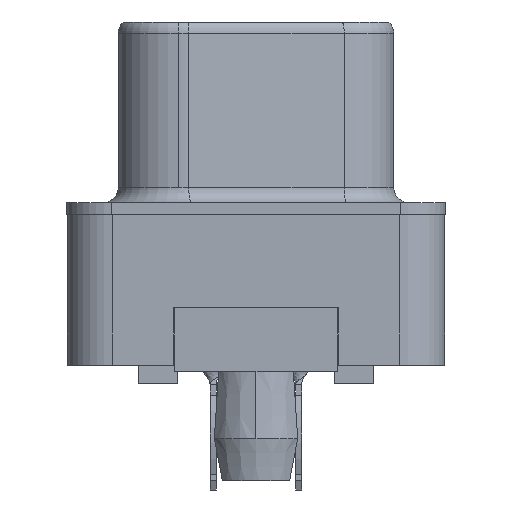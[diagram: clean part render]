
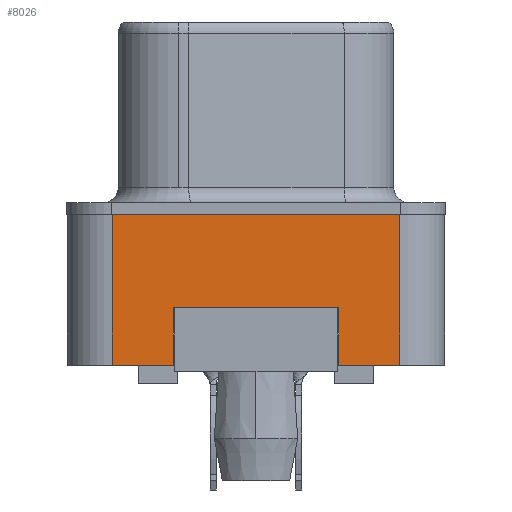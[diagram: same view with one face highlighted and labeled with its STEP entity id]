
A CAD part, left-side view. The second image highlights one B-rep face of the part: STEP entity #8026.
In plain terms, the highlighted planar face has unit normal (-1, 0, 0).
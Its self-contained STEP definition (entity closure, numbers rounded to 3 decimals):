
#513 = DIRECTION ( 'NONE',  ( 0., -1., 0. ) ) ;
#1822 = VECTOR ( 'NONE', #6721, 1000. ) ;
#1927 = LINE ( 'NONE', #18208, #1822 ) ;
#1981 = DIRECTION ( 'NONE',  ( 0., 0., 1. ) ) ;
#2326 = CARTESIAN_POINT ( 'NONE',  ( -2.91, -4.775, -5. ) ) ;
#2672 = ORIENTED_EDGE ( 'NONE', *, *, #16498, .T. ) ;
#4367 = VERTEX_POINT ( 'NONE', #11320 ) ;
#4892 = ORIENTED_EDGE ( 'NONE', *, *, #25048, .T. ) ;
#5143 = CARTESIAN_POINT ( 'NONE',  ( -2.91, 4.775, -5. ) ) ;
#5701 = CARTESIAN_POINT ( 'NONE',  ( -2.91, -2.75, -3.1 ) ) ;
#5786 = FACE_OUTER_BOUND ( 'NONE', #18704, .T. ) ;
#6436 = DIRECTION ( 'NONE',  ( 0., 0., -1. ) ) ;
#6721 = DIRECTION ( 'NONE',  ( 0., 1., 0. ) ) ;
#6991 = CARTESIAN_POINT ( 'NONE',  ( -2.91, 4.775, 0. ) ) ;
#7466 = VERTEX_POINT ( 'NONE', #18600 ) ;
#7940 = ORIENTED_EDGE ( 'NONE', *, *, #27114, .T. ) ;
#8026 = ADVANCED_FACE ( 'NONE', ( #5786 ), #14947, .T. ) ;
#8445 = EDGE_CURVE ( 'NONE', #7466, #29047, #26905, .T. ) ;
#9882 = CARTESIAN_POINT ( 'NONE',  ( -2.91, 2.75, -5. ) ) ;
#11117 = CARTESIAN_POINT ( 'NONE',  ( -2.91, -4.775, -5. ) ) ;
#11320 = CARTESIAN_POINT ( 'NONE',  ( -2.91, -4.775, 0. ) ) ;
#11336 = ORIENTED_EDGE ( 'NONE', *, *, #18535, .F. ) ;
#12314 = CARTESIAN_POINT ( 'NONE',  ( -2.91, -2.75, -5. ) ) ;
#12468 = CARTESIAN_POINT ( 'NONE',  ( -2.91, -4.775, -5. ) ) ;
#12479 = VERTEX_POINT ( 'NONE', #12314 ) ;
#12763 = VERTEX_POINT ( 'NONE', #6991 ) ;
#13031 = ORIENTED_EDGE ( 'NONE', *, *, #29729, .F. ) ;
#13086 = ORIENTED_EDGE ( 'NONE', *, *, #8445, .F. ) ;
#14098 = LINE ( 'NONE', #2326, #21895 ) ;
#14415 = LINE ( 'NONE', #23556, #16154 ) ;
#14947 = PLANE ( 'NONE',  #27943 ) ;
#15477 = VECTOR ( 'NONE', #29035, 1000. ) ;
#16154 = VECTOR ( 'NONE', #19357, 1000. ) ;
#16337 = VERTEX_POINT ( 'NONE', #27277 ) ;
#16498 = EDGE_CURVE ( 'NONE', #12479, #27361, #14098, .T. ) ;
#17266 = CARTESIAN_POINT ( 'NONE',  ( -2.91, -4.775, 0. ) ) ;
#17276 = DIRECTION ( 'NONE',  ( 0., 0., 1. ) ) ;
#17309 = DIRECTION ( 'NONE',  ( 0., 0., -1. ) ) ;
#17540 = VECTOR ( 'NONE', #6436, 1000. ) ;
#17584 = EDGE_CURVE ( 'NONE', #12763, #4367, #19580, .T. ) ;
#18208 = CARTESIAN_POINT ( 'NONE',  ( -2.91, 2.75, -3.1 ) ) ;
#18535 = EDGE_CURVE ( 'NONE', #16337, #12763, #26393, .T. ) ;
#18600 = CARTESIAN_POINT ( 'NONE',  ( -2.91, 2.75, -3.1 ) ) ;
#18704 = EDGE_LOOP ( 'NONE', ( #7940, #2672, #25230, #27100, #11336, #4892, #13086, #13031 ) ) ;
#19357 = DIRECTION ( 'NONE',  ( 0., -1., 0. ) ) ;
#19580 = LINE ( 'NONE', #17266, #30292 ) ;
#20697 = CARTESIAN_POINT ( 'NONE',  ( -2.91, -2.75, -3.1 ) ) ;
#21360 = DIRECTION ( 'NONE',  ( 0., -1., 0. ) ) ;
#21895 = VECTOR ( 'NONE', #21360, 1000. ) ;
#23556 = CARTESIAN_POINT ( 'NONE',  ( -2.91, -4.775, -5. ) ) ;
#25048 = EDGE_CURVE ( 'NONE', #16337, #29047, #14415, .T. ) ;
#25230 = ORIENTED_EDGE ( 'NONE', *, *, #26553, .T. ) ;
#25431 = VECTOR ( 'NONE', #1981, 1000. ) ;
#26393 = LINE ( 'NONE', #5143, #15477 ) ;
#26502 = VERTEX_POINT ( 'NONE', #5701 ) ;
#26553 = EDGE_CURVE ( 'NONE', #27361, #4367, #30509, .T. ) ;
#26905 = LINE ( 'NONE', #29394, #28474 ) ;
#27027 = DIRECTION ( 'NONE',  ( -1., 0., 0. ) ) ;
#27100 = ORIENTED_EDGE ( 'NONE', *, *, #17584, .F. ) ;
#27114 = EDGE_CURVE ( 'NONE', #26502, #12479, #27834, .T. ) ;
#27277 = CARTESIAN_POINT ( 'NONE',  ( -2.91, 4.775, -5. ) ) ;
#27361 = VERTEX_POINT ( 'NONE', #28576 ) ;
#27834 = LINE ( 'NONE', #20697, #17540 ) ;
#27943 = AXIS2_PLACEMENT_3D ( 'NONE', #12468, #27027, #17276 ) ;
#28474 = VECTOR ( 'NONE', #17309, 1000. ) ;
#28576 = CARTESIAN_POINT ( 'NONE',  ( -2.91, -4.775, -5. ) ) ;
#29035 = DIRECTION ( 'NONE',  ( 0., 0., 1. ) ) ;
#29047 = VERTEX_POINT ( 'NONE', #9882 ) ;
#29394 = CARTESIAN_POINT ( 'NONE',  ( -2.91, 2.75, -3.1 ) ) ;
#29729 = EDGE_CURVE ( 'NONE', #26502, #7466, #1927, .T. ) ;
#30292 = VECTOR ( 'NONE', #513, 1000. ) ;
#30509 = LINE ( 'NONE', #11117, #25431 ) ;
